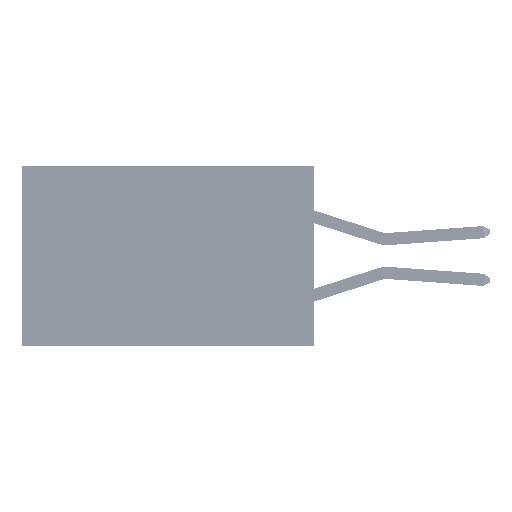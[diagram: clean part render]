
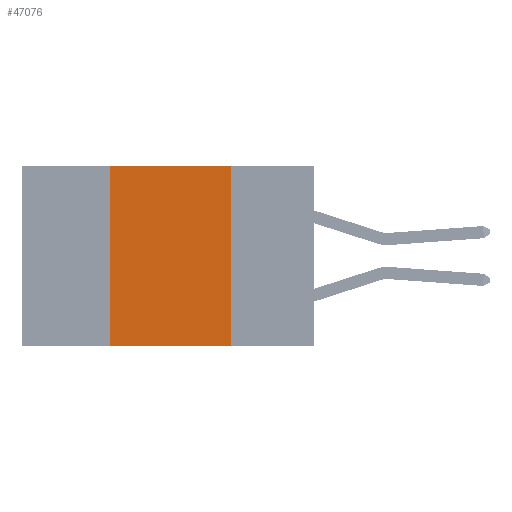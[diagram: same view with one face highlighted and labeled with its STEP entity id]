
A CAD part, left-side view. The second image highlights one B-rep face of the part: STEP entity #47076.
In plain terms, the highlighted planar face has unit normal (-1, 0, 0).
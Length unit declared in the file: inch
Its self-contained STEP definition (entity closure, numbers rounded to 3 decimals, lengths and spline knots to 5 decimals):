
#1090 = ORIENTED_EDGE ( 'NONE', *, *, #1170, .F. ) ;
#1170 = EDGE_CURVE ( 'NONE', #32694, #21546, #34988, .T. ) ;
#2447 = LINE ( 'NONE', #18349, #26014 ) ;
#3044 = DIRECTION ( 'NONE',  ( 0., 0., -1. ) ) ;
#4774 = ORIENTED_EDGE ( 'NONE', *, *, #41270, .T. ) ;
#6129 = CARTESIAN_POINT ( 'NONE',  ( 0., 0.42, 0. ) ) ;
#7514 = VECTOR ( 'NONE', #39893, 39.37008 ) ;
#8367 = EDGE_LOOP ( 'NONE', ( #34586, #1090, #27135, #4774 ) ) ;
#9144 = CARTESIAN_POINT ( 'NONE',  ( 0., 0.17, 0. ) ) ;
#11770 = VECTOR ( 'NONE', #36566, 39.37008 ) ;
#14633 = DIRECTION ( 'NONE',  ( 0., -1., 0. ) ) ;
#14782 = CARTESIAN_POINT ( 'NONE',  ( 0., 0.17, 0. ) ) ;
#17838 = CARTESIAN_POINT ( 'NONE',  ( 0., 0.6, 0. ) ) ;
#18349 = CARTESIAN_POINT ( 'NONE',  ( 0., 0.6, -0.37 ) ) ;
#19806 = VECTOR ( 'NONE', #31480, 39.37008 ) ;
#21546 = VERTEX_POINT ( 'NONE', #9144 ) ;
#26014 = VECTOR ( 'NONE', #14633, 39.37008 ) ;
#27135 = ORIENTED_EDGE ( 'NONE', *, *, #46409, .F. ) ;
#28678 = CARTESIAN_POINT ( 'NONE',  ( 0., 0.6, 0. ) ) ;
#28974 = LINE ( 'NONE', #14782, #11770 ) ;
#29533 = CARTESIAN_POINT ( 'NONE',  ( 0., 0.42, -0.37 ) ) ;
#30689 = EDGE_CURVE ( 'NONE', #21546, #38385, #28974, .T. ) ;
#31480 = DIRECTION ( 'NONE',  ( 0., 0., 1. ) ) ;
#32694 = VERTEX_POINT ( 'NONE', #6129 ) ;
#34586 = ORIENTED_EDGE ( 'NONE', *, *, #30689, .F. ) ;
#34988 = LINE ( 'NONE', #28678, #7514 ) ;
#36389 = PLANE ( 'NONE',  #40563 ) ;
#36566 = DIRECTION ( 'NONE',  ( 0., 0., -1. ) ) ;
#37080 = CARTESIAN_POINT ( 'NONE',  ( 0., 0.17, -0.37 ) ) ;
#38385 = VERTEX_POINT ( 'NONE', #37080 ) ;
#39874 = LINE ( 'NONE', #43155, #19806 ) ;
#39893 = DIRECTION ( 'NONE',  ( 0., -1., 0. ) ) ;
#40563 = AXIS2_PLACEMENT_3D ( 'NONE', #17838, #43769, #3044 ) ;
#41270 = EDGE_CURVE ( 'NONE', #43655, #38385, #2447, .T. ) ;
#43155 = CARTESIAN_POINT ( 'NONE',  ( 0., 0.42, 0. ) ) ;
#43655 = VERTEX_POINT ( 'NONE', #29533 ) ;
#43769 = DIRECTION ( 'NONE',  ( 1., 0., 0. ) ) ;
#45939 = FACE_OUTER_BOUND ( 'NONE', #8367, .T. ) ;
#46409 = EDGE_CURVE ( 'NONE', #43655, #32694, #39874, .T. ) ;
#47076 = ADVANCED_FACE ( 'NONE', ( #45939 ), #36389, .F. ) ;
